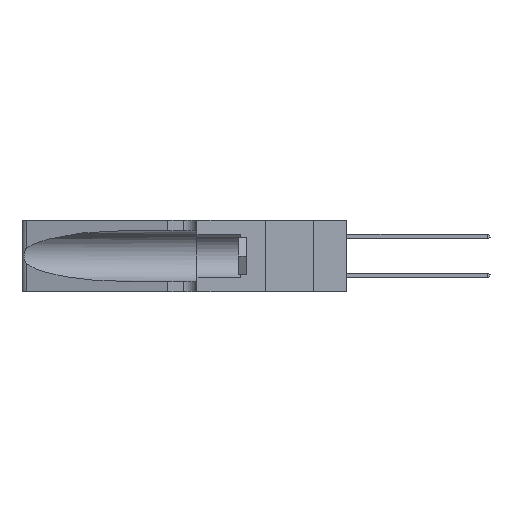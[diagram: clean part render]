
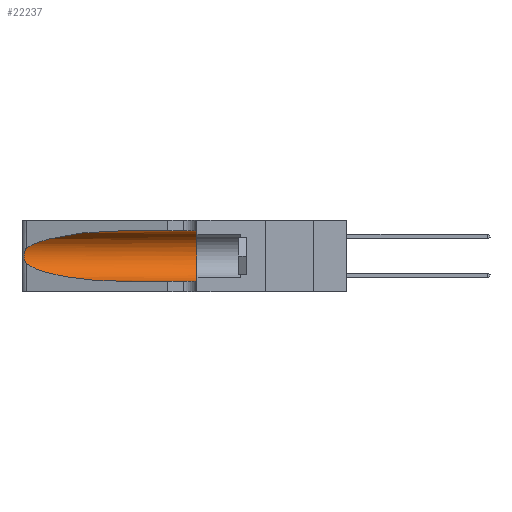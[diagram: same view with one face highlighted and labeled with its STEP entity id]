
A CAD part, left-side view. The second image highlights one B-rep face of the part: STEP entity #22237.
In plain terms, the highlighted cylindrical face has radius 3.308 mm (diameter 6.617 mm), a partial arc.
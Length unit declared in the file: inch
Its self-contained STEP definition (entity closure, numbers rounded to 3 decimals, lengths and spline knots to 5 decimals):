
#133 = DIRECTION ( 'NONE',  ( 0., 0., -1. ) ) ;
#259 = CARTESIAN_POINT ( 'NONE',  ( 0.25487, 1.22718, 0.22369 ) ) ;
#1869 = VECTOR ( 'NONE', #16636, 39.37008 ) ;
#1896 = VERTEX_POINT ( 'NONE', #27987 ) ;
#2041 = VERTEX_POINT ( 'NONE', #3384 ) ;
#2068 = EDGE_CURVE ( 'NONE', #2041, #18418, #7770, .T. ) ;
#2076 = CARTESIAN_POINT ( 'NONE',  ( 0.25555, 1.22993, 0.14849 ) ) ;
#2463 =( BOUNDED_CURVE ( )  B_SPLINE_CURVE ( 3, ( #15436, #3816, #20093, #6198 ),
 .UNSPECIFIED., .F., .T. ) 
 B_SPLINE_CURVE_WITH_KNOTS ( ( 4, 4 ),
 ( 3.44316, 4.71239 ),
 .UNSPECIFIED. ) 
 CURVE ( )  GEOMETRIC_REPRESENTATION_ITEM ( )  RATIONAL_B_SPLINE_CURVE ( ( 1., 0.87, 0.87, 1. ) ) 
 REPRESENTATION_ITEM ( '' )  );
#2552 = CARTESIAN_POINT ( 'NONE',  ( 0.18966, 0.96281, 0.31525 ) ) ;
#2560 = CARTESIAN_POINT ( 'NONE',  ( 0.1305, 1.61858, 0.05475 ) ) ;
#2887 = CARTESIAN_POINT ( 'NONE',  ( 0.25555, 1.22994, 0.2215 ) ) ;
#3384 = CARTESIAN_POINT ( 'NONE',  ( 0.25487, 1.22718, 0.22369 ) ) ;
#3621 = EDGE_CURVE ( 'NONE', #23475, #1896, #20475, .T. ) ;
#3762 = DIRECTION ( 'NONE',  ( 0., 1., 0. ) ) ;
#3816 = CARTESIAN_POINT ( 'NONE',  ( 0.2373, 1.15595, 0.08982 ) ) ;
#4904 = DIRECTION ( 'NONE',  ( 0., -1., 0. ) ) ;
#6119 = CARTESIAN_POINT ( 'NONE',  ( 0.25787, 1.23484, 0.2124 ) ) ;
#6198 = CARTESIAN_POINT ( 'NONE',  ( 0.1305, 0.72297, 0.05475 ) ) ;
#7559 = VECTOR ( 'NONE', #20259, 39.37008 ) ;
#7573 = CARTESIAN_POINT ( 'NONE',  ( 0.25639, 1.23186, 0.15144 ) ) ;
#7619 = EDGE_CURVE ( 'NONE', #23241, #1896, #15566, .T. ) ;
#7770 = B_SPLINE_CURVE_WITH_KNOTS ( 'NONE', 3,
 ( #8753, #2887, #16964, #6119, #23215, #23421, #26348, #23951, #16670, #19390, #10495, #7573, #2076, #14913 ),
 .UNSPECIFIED., .F., .F.,
 ( 4, 2, 2, 2, 2, 2, 4 ),
 ( 0., 0.00027, 0.00053, 0.00107, 0.0016, 0.00187, 0.00214 ),
 .UNSPECIFIED. ) ;
#7885 =( BOUNDED_CURVE ( )  B_SPLINE_CURVE ( 3, ( #9639, #2552, #14301, #259 ),
 .UNSPECIFIED., .F., .F. ) 
 B_SPLINE_CURVE_WITH_KNOTS ( ( 4, 4 ),
 ( 1.5708, 2.84003 ),
 .UNSPECIFIED. ) 
 CURVE ( )  GEOMETRIC_REPRESENTATION_ITEM ( )  RATIONAL_B_SPLINE_CURVE ( ( 1., 0.87, 0.87, 1. ) ) 
 REPRESENTATION_ITEM ( '' )  );
#8753 = CARTESIAN_POINT ( 'NONE',  ( 0.25487, 1.22718, 0.22369 ) ) ;
#8773 = VERTEX_POINT ( 'NONE', #13697 ) ;
#8915 = FACE_OUTER_BOUND ( 'NONE', #17950, .T. ) ;
#9639 = CARTESIAN_POINT ( 'NONE',  ( 0.1305, 0.72297, 0.31525 ) ) ;
#10495 = CARTESIAN_POINT ( 'NONE',  ( 0.25789, 1.23486, 0.15765 ) ) ;
#11575 = AXIS2_PLACEMENT_3D ( 'NONE', #18826, #4904, #133 ) ;
#11614 = EDGE_CURVE ( 'NONE', #8773, #2041, #7885, .T. ) ;
#12065 = ORIENTED_EDGE ( 'NONE', *, *, #20757, .T. ) ;
#13697 = CARTESIAN_POINT ( 'NONE',  ( 0.1305, 0.72297, 0.31525 ) ) ;
#14301 = CARTESIAN_POINT ( 'NONE',  ( 0.2373, 1.15595, 0.28018 ) ) ;
#14913 = CARTESIAN_POINT ( 'NONE',  ( 0.25487, 1.22718, 0.14631 ) ) ;
#15436 = CARTESIAN_POINT ( 'NONE',  ( 0.25487, 1.22718, 0.14631 ) ) ;
#15566 = CIRCLE ( 'NONE', #19342, 0.13025 ) ;
#16636 = DIRECTION ( 'NONE',  ( 0., -1., 0. ) ) ;
#16670 = CARTESIAN_POINT ( 'NONE',  ( 0.26017, 1.23833, 0.17102 ) ) ;
#16962 = ORIENTED_EDGE ( 'NONE', *, *, #28054, .F. ) ;
#16964 = CARTESIAN_POINT ( 'NONE',  ( 0.25639, 1.23184, 0.21858 ) ) ;
#17714 = CARTESIAN_POINT ( 'NONE',  ( 0.1305, 0.35, 0.185 ) ) ;
#17921 = CARTESIAN_POINT ( 'NONE',  ( 0.1305, 1.61858, 0.31525 ) ) ;
#17950 = EDGE_LOOP ( 'NONE', ( #25394, #19776, #12065, #28676, #20704, #16962 ) ) ;
#18418 = VERTEX_POINT ( 'NONE', #25548 ) ;
#18434 = LINE ( 'NONE', #17921, #7559 ) ;
#18826 = CARTESIAN_POINT ( 'NONE',  ( 0.1305, 1.61858, 0.185 ) ) ;
#19342 = AXIS2_PLACEMENT_3D ( 'NONE', #17714, #3762, #20051 ) ;
#19390 = CARTESIAN_POINT ( 'NONE',  ( 0.25856, 1.23593, 0.16098 ) ) ;
#19776 = ORIENTED_EDGE ( 'NONE', *, *, #2068, .T. ) ;
#19874 = CARTESIAN_POINT ( 'NONE',  ( 0.1305, 0.35, 0.31525 ) ) ;
#20051 = DIRECTION ( 'NONE',  ( 0., 0., 1. ) ) ;
#20093 = CARTESIAN_POINT ( 'NONE',  ( 0.18966, 0.96281, 0.05475 ) ) ;
#20259 = DIRECTION ( 'NONE',  ( 0., -1., 0. ) ) ;
#20475 = LINE ( 'NONE', #2560, #1869 ) ;
#20704 = ORIENTED_EDGE ( 'NONE', *, *, #7619, .F. ) ;
#20757 = EDGE_CURVE ( 'NONE', #18418, #23475, #2463, .T. ) ;
#22237 = ADVANCED_FACE ( 'NONE', ( #8915 ), #26530, .F. ) ;
#23215 = CARTESIAN_POINT ( 'NONE',  ( 0.25854, 1.2359, 0.20912 ) ) ;
#23241 = VERTEX_POINT ( 'NONE', #19874 ) ;
#23421 = CARTESIAN_POINT ( 'NONE',  ( 0.26018, 1.23835, 0.19895 ) ) ;
#23475 = VERTEX_POINT ( 'NONE', #29715 ) ;
#23951 = CARTESIAN_POINT ( 'NONE',  ( 0.26075, 1.23896, 0.178 ) ) ;
#25394 = ORIENTED_EDGE ( 'NONE', *, *, #11614, .T. ) ;
#25548 = CARTESIAN_POINT ( 'NONE',  ( 0.25487, 1.22718, 0.14631 ) ) ;
#26348 = CARTESIAN_POINT ( 'NONE',  ( 0.26075, 1.23896, 0.19203 ) ) ;
#26530 = CYLINDRICAL_SURFACE ( 'NONE', #11575, 0.13025 ) ;
#27987 = CARTESIAN_POINT ( 'NONE',  ( 0.1305, 0.35, 0.05475 ) ) ;
#28054 = EDGE_CURVE ( 'NONE', #8773, #23241, #18434, .T. ) ;
#28676 = ORIENTED_EDGE ( 'NONE', *, *, #3621, .T. ) ;
#29715 = CARTESIAN_POINT ( 'NONE',  ( 0.1305, 0.72297, 0.05475 ) ) ;
